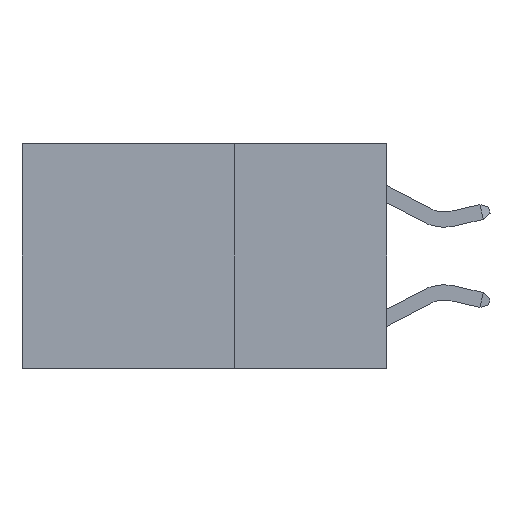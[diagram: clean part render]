
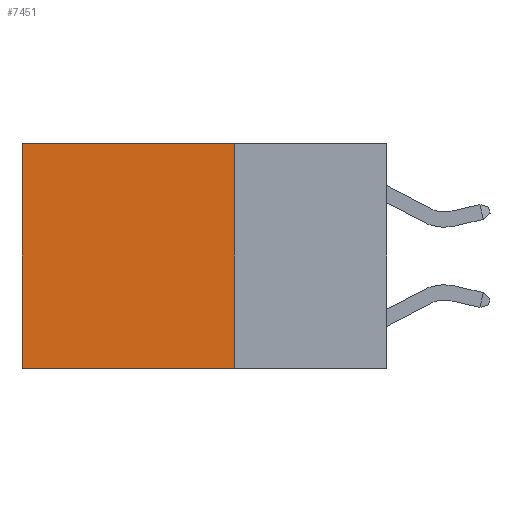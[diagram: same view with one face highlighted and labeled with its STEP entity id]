
A CAD part, left-side view. The second image highlights one B-rep face of the part: STEP entity #7451.
In plain terms, the highlighted planar face has unit normal (-1, 0, 0).
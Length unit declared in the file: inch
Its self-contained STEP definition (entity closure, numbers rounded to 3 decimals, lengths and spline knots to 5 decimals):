
#170 = VERTEX_POINT ( 'NONE', #5059 ) ;
#325 = ORIENTED_EDGE ( 'NONE', *, *, #5607, .T. ) ;
#547 = VECTOR ( 'NONE', #4834, 39.37008 ) ;
#784 = CARTESIAN_POINT ( 'NONE',  ( 0.2625, 0.6, 0. ) ) ;
#960 = DIRECTION ( 'NONE',  ( 1., 0., 0. ) ) ;
#1490 = EDGE_CURVE ( 'NONE', #5597, #170, #2623, .T. ) ;
#1874 = VECTOR ( 'NONE', #7688, 39.37008 ) ;
#2006 = DIRECTION ( 'NONE',  ( 0., 1., 0. ) ) ;
#2623 = LINE ( 'NONE', #784, #547 ) ;
#3121 = ORIENTED_EDGE ( 'NONE', *, *, #1490, .T. ) ;
#3181 = CARTESIAN_POINT ( 'NONE',  ( 0.2625, 0.25, 0. ) ) ;
#3345 = LINE ( 'NONE', #5245, #6961 ) ;
#3702 = CARTESIAN_POINT ( 'NONE',  ( 0.2625, 0.25, 0. ) ) ;
#3819 = CARTESIAN_POINT ( 'NONE',  ( 0.2625, 0.6, 0. ) ) ;
#3856 = LINE ( 'NONE', #3181, #7228 ) ;
#3974 = EDGE_LOOP ( 'NONE', ( #3121, #6374, #7906, #325 ) ) ;
#4119 = CARTESIAN_POINT ( 'NONE',  ( 0.2625, 0.25, 0. ) ) ;
#4262 = PLANE ( 'NONE',  #4662 ) ;
#4662 = AXIS2_PLACEMENT_3D ( 'NONE', #6886, #960, #6246 ) ;
#4736 = EDGE_CURVE ( 'NONE', #7264, #170, #3345, .T. ) ;
#4834 = DIRECTION ( 'NONE',  ( 0., 0., -1. ) ) ;
#4890 = CARTESIAN_POINT ( 'NONE',  ( 0.2625, 0.25, -0.37 ) ) ;
#5051 = LINE ( 'NONE', #3702, #1874 ) ;
#5059 = CARTESIAN_POINT ( 'NONE',  ( 0.2625, 0.6, -0.37 ) ) ;
#5245 = CARTESIAN_POINT ( 'NONE',  ( 0.2625, 0.25, -0.37 ) ) ;
#5597 = VERTEX_POINT ( 'NONE', #3819 ) ;
#5607 = EDGE_CURVE ( 'NONE', #7623, #5597, #3856, .T. ) ;
#5818 = DIRECTION ( 'NONE',  ( 0., 1., 0. ) ) ;
#5819 = EDGE_CURVE ( 'NONE', #7623, #7264, #5051, .T. ) ;
#6246 = DIRECTION ( 'NONE',  ( 0., 0., -1. ) ) ;
#6374 = ORIENTED_EDGE ( 'NONE', *, *, #4736, .F. ) ;
#6886 = CARTESIAN_POINT ( 'NONE',  ( 0.2625, 0.25, 0. ) ) ;
#6961 = VECTOR ( 'NONE', #2006, 39.37008 ) ;
#7228 = VECTOR ( 'NONE', #5818, 39.37008 ) ;
#7264 = VERTEX_POINT ( 'NONE', #4890 ) ;
#7451 = ADVANCED_FACE ( 'NONE', ( #7527 ), #4262, .F. ) ;
#7527 = FACE_OUTER_BOUND ( 'NONE', #3974, .T. ) ;
#7623 = VERTEX_POINT ( 'NONE', #4119 ) ;
#7688 = DIRECTION ( 'NONE',  ( 0., 0., -1. ) ) ;
#7906 = ORIENTED_EDGE ( 'NONE', *, *, #5819, .F. ) ;
